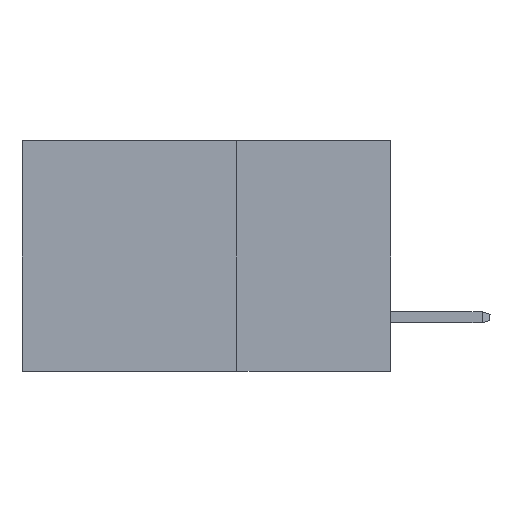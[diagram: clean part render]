
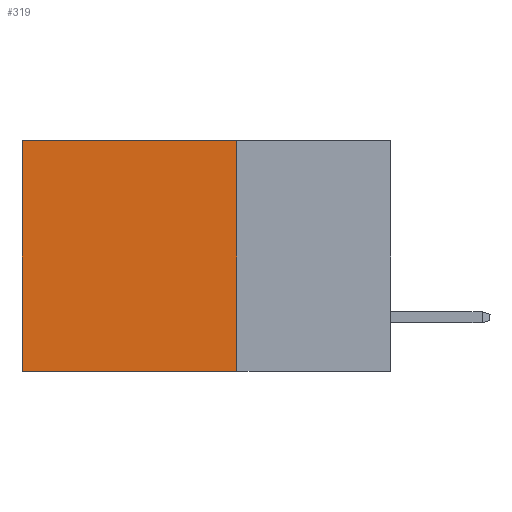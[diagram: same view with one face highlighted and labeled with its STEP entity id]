
A CAD part, left-side view. The second image highlights one B-rep face of the part: STEP entity #319.
In plain terms, the highlighted planar face has unit normal (-1, 0, 0).
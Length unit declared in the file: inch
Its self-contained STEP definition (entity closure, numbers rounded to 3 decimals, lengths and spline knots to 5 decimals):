
#319 = ADVANCED_FACE ( 'NONE', ( #2705 ), #1317, .F. ) ;
#1132 = VERTEX_POINT ( 'NONE', #8426 ) ;
#1258 = DIRECTION ( 'NONE',  ( 0., 0., -1. ) ) ;
#1317 = PLANE ( 'NONE',  #7171 ) ;
#1784 = EDGE_CURVE ( 'NONE', #6372, #7845, #7450, .T. ) ;
#2040 = ORIENTED_EDGE ( 'NONE', *, *, #3596, .T. ) ;
#2270 = CARTESIAN_POINT ( 'NONE',  ( 0.2875, 0.25, -0.375 ) ) ;
#2705 = FACE_OUTER_BOUND ( 'NONE', #12525, .T. ) ;
#2788 = ORIENTED_EDGE ( 'NONE', *, *, #5581, .F. ) ;
#3292 = DIRECTION ( 'NONE',  ( 0., 1., 0. ) ) ;
#3596 = EDGE_CURVE ( 'NONE', #7845, #9323, #12387, .T. ) ;
#3597 = LINE ( 'NONE', #11267, #4837 ) ;
#4579 = DIRECTION ( 'NONE',  ( 0., 0., -1. ) ) ;
#4837 = VECTOR ( 'NONE', #1258, 39.37008 ) ;
#5581 = EDGE_CURVE ( 'NONE', #6372, #1132, #3597, .T. ) ;
#5906 = CARTESIAN_POINT ( 'NONE',  ( 0.2875, 0.6, 0. ) ) ;
#6014 = EDGE_CURVE ( 'NONE', #1132, #9323, #13288, .T. ) ;
#6372 = VERTEX_POINT ( 'NONE', #9918 ) ;
#7161 = CARTESIAN_POINT ( 'NONE',  ( 0.2875, 0.25, -0.375 ) ) ;
#7171 = AXIS2_PLACEMENT_3D ( 'NONE', #7161, #12775, #11614 ) ;
#7305 = CARTESIAN_POINT ( 'NONE',  ( 0.2875, 0.25, 0. ) ) ;
#7450 = LINE ( 'NONE', #7305, #9780 ) ;
#7845 = VERTEX_POINT ( 'NONE', #5906 ) ;
#8426 = CARTESIAN_POINT ( 'NONE',  ( 0.2875, 0.25, -0.375 ) ) ;
#9323 = VERTEX_POINT ( 'NONE', #13567 ) ;
#9444 = CARTESIAN_POINT ( 'NONE',  ( 0.2875, 0.6, -0.375 ) ) ;
#9780 = VECTOR ( 'NONE', #13067, 39.37008 ) ;
#9918 = CARTESIAN_POINT ( 'NONE',  ( 0.2875, 0.25, 0. ) ) ;
#9927 = ORIENTED_EDGE ( 'NONE', *, *, #1784, .T. ) ;
#10594 = VECTOR ( 'NONE', #4579, 39.37008 ) ;
#10681 = VECTOR ( 'NONE', #3292, 39.37008 ) ;
#11267 = CARTESIAN_POINT ( 'NONE',  ( 0.2875, 0.25, -0.375 ) ) ;
#11614 = DIRECTION ( 'NONE',  ( 0., 0., -1. ) ) ;
#12387 = LINE ( 'NONE', #9444, #10594 ) ;
#12525 = EDGE_LOOP ( 'NONE', ( #2040, #13335, #2788, #9927 ) ) ;
#12775 = DIRECTION ( 'NONE',  ( 1., 0., 0. ) ) ;
#13067 = DIRECTION ( 'NONE',  ( 0., 1., 0. ) ) ;
#13288 = LINE ( 'NONE', #2270, #10681 ) ;
#13335 = ORIENTED_EDGE ( 'NONE', *, *, #6014, .F. ) ;
#13567 = CARTESIAN_POINT ( 'NONE',  ( 0.2875, 0.6, -0.375 ) ) ;
